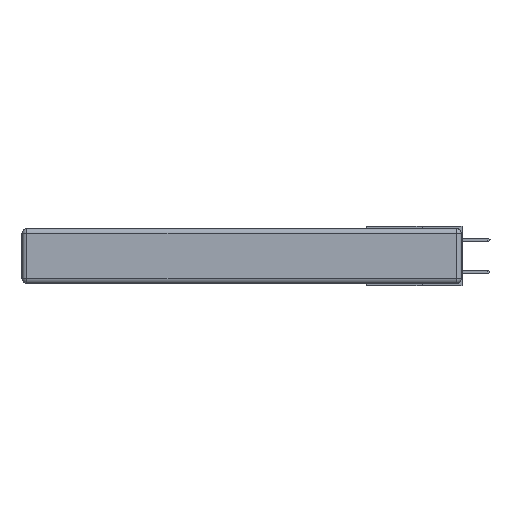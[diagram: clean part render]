
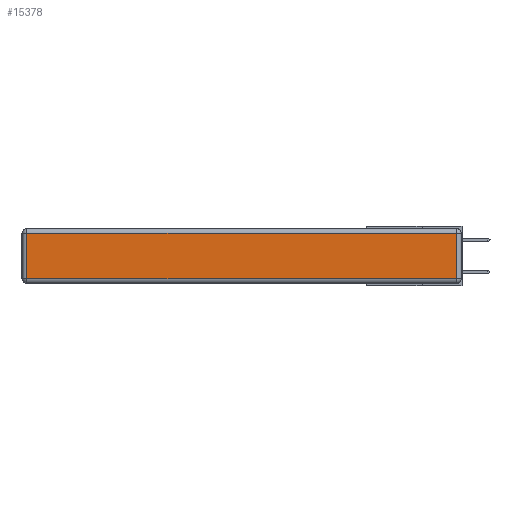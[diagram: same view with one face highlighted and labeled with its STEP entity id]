
A CAD part, left-side view. The second image highlights one B-rep face of the part: STEP entity #15378.
In plain terms, the highlighted planar face has unit normal (-1, 0, 0).
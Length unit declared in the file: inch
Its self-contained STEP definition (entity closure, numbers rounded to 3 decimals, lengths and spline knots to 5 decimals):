
#1280 = LINE ( 'NONE', #15677, #22682 ) ;
#2874 = FACE_OUTER_BOUND ( 'NONE', #6440, .T. ) ;
#3797 = CARTESIAN_POINT ( 'NONE',  ( 0., 0.03, -0.313 ) ) ;
#6440 = EDGE_LOOP ( 'NONE', ( #17386, #9319, #29587, #14512 ) ) ;
#6636 = EDGE_CURVE ( 'NONE', #21009, #15370, #24066, .T. ) ;
#7141 = LINE ( 'NONE', #29203, #32764 ) ;
#7784 = EDGE_CURVE ( 'NONE', #19441, #21009, #1280, .T. ) ;
#8144 = DIRECTION ( 'NONE',  ( -1., 0., 0. ) ) ;
#9319 = ORIENTED_EDGE ( 'NONE', *, *, #19939, .T. ) ;
#9536 = VECTOR ( 'NONE', #35065, 39.37008 ) ;
#12523 = VERTEX_POINT ( 'NONE', #3797 ) ;
#13252 = CARTESIAN_POINT ( 'NONE',  ( 0., 2.72, -0.313 ) ) ;
#14061 = CARTESIAN_POINT ( 'NONE',  ( 0., 0.03, -0.03 ) ) ;
#14512 = ORIENTED_EDGE ( 'NONE', *, *, #6636, .T. ) ;
#15370 = VERTEX_POINT ( 'NONE', #13252 ) ;
#15378 = ADVANCED_FACE ( 'NONE', ( #2874 ), #16345, .T. ) ;
#15677 = CARTESIAN_POINT ( 'NONE',  ( 0., 2.75, -0.03 ) ) ;
#16249 = DIRECTION ( 'NONE',  ( 0., 0., 1. ) ) ;
#16345 = PLANE ( 'NONE',  #18741 ) ;
#17386 = ORIENTED_EDGE ( 'NONE', *, *, #19123, .T. ) ;
#17884 = VECTOR ( 'NONE', #20269, 39.37008 ) ;
#18741 = AXIS2_PLACEMENT_3D ( 'NONE', #32385, #8144, #16249 ) ;
#19123 = EDGE_CURVE ( 'NONE', #15370, #12523, #24701, .T. ) ;
#19441 = VERTEX_POINT ( 'NONE', #14061 ) ;
#19939 = EDGE_CURVE ( 'NONE', #12523, #19441, #7141, .T. ) ;
#20269 = DIRECTION ( 'NONE',  ( 0., -1., 0. ) ) ;
#21009 = VERTEX_POINT ( 'NONE', #25784 ) ;
#21387 = CARTESIAN_POINT ( 'NONE',  ( 0., 2.72, -0.343 ) ) ;
#22682 = VECTOR ( 'NONE', #32180, 39.37008 ) ;
#24066 = LINE ( 'NONE', #21387, #9536 ) ;
#24701 = LINE ( 'NONE', #28769, #17884 ) ;
#25784 = CARTESIAN_POINT ( 'NONE',  ( 0., 2.72, -0.03 ) ) ;
#28769 = CARTESIAN_POINT ( 'NONE',  ( 0., 0., -0.313 ) ) ;
#29203 = CARTESIAN_POINT ( 'NONE',  ( 0., 0.03, -0.343 ) ) ;
#29587 = ORIENTED_EDGE ( 'NONE', *, *, #7784, .T. ) ;
#32180 = DIRECTION ( 'NONE',  ( 0., 1., 0. ) ) ;
#32385 = CARTESIAN_POINT ( 'NONE',  ( 0., 0., -0.343 ) ) ;
#32764 = VECTOR ( 'NONE', #34709, 39.37008 ) ;
#34709 = DIRECTION ( 'NONE',  ( 0., 0., 1. ) ) ;
#35065 = DIRECTION ( 'NONE',  ( 0., 0., -1. ) ) ;
